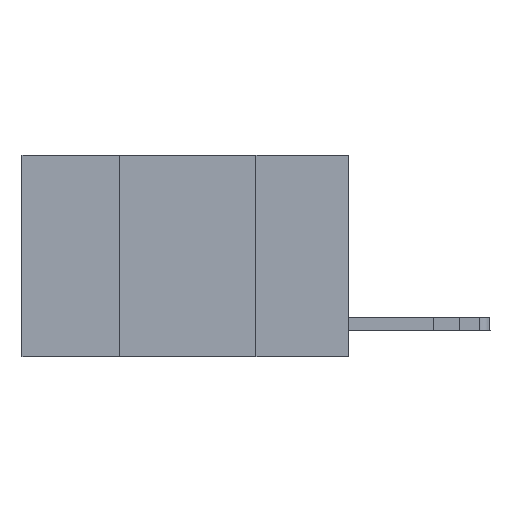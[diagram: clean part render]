
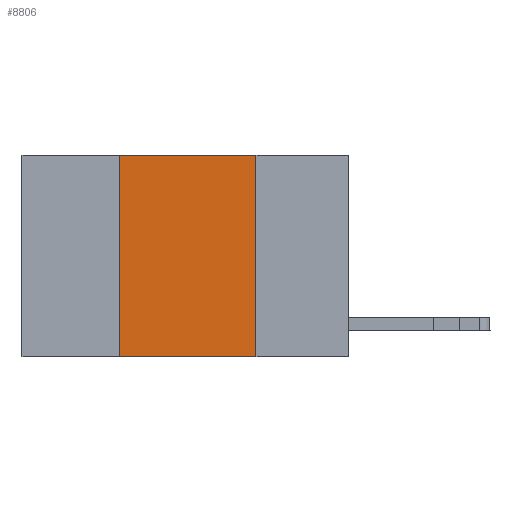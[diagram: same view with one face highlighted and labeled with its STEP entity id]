
A CAD part, left-side view. The second image highlights one B-rep face of the part: STEP entity #8806.
In plain terms, the highlighted planar face has unit normal (-1, 0, 0).
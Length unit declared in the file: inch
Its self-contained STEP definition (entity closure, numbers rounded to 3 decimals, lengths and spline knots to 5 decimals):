
#1164 = EDGE_CURVE ( 'NONE', #3525, #4443, #15752, .T. ) ;
#1372 = VECTOR ( 'NONE', #15229, 39.37008 ) ;
#1936 = LINE ( 'NONE', #8537, #1372 ) ;
#2475 = CARTESIAN_POINT ( 'NONE',  ( 0., 0.17, -0.37 ) ) ;
#3525 = VERTEX_POINT ( 'NONE', #12645 ) ;
#3609 = PLANE ( 'NONE',  #5714 ) ;
#3705 = DIRECTION ( 'NONE',  ( 1., 0., 0. ) ) ;
#3741 = CARTESIAN_POINT ( 'NONE',  ( 0., 0.17, 0. ) ) ;
#4443 = VERTEX_POINT ( 'NONE', #2475 ) ;
#5211 = VECTOR ( 'NONE', #13344, 39.37008 ) ;
#5714 = AXIS2_PLACEMENT_3D ( 'NONE', #7008, #3705, #20737 ) ;
#7008 = CARTESIAN_POINT ( 'NONE',  ( 0., 0.6, 0. ) ) ;
#7611 = ORIENTED_EDGE ( 'NONE', *, *, #21292, .F. ) ;
#7775 = DIRECTION ( 'NONE',  ( 0., -1., 0. ) ) ;
#7928 = VERTEX_POINT ( 'NONE', #10378 ) ;
#8105 = ORIENTED_EDGE ( 'NONE', *, *, #1164, .F. ) ;
#8537 = CARTESIAN_POINT ( 'NONE',  ( 0., 0.6, -0.37 ) ) ;
#8554 = FACE_OUTER_BOUND ( 'NONE', #21101, .T. ) ;
#8806 = ADVANCED_FACE ( 'NONE', ( #8554 ), #3609, .F. ) ;
#8843 = CARTESIAN_POINT ( 'NONE',  ( 0., 0.42, 0. ) ) ;
#10378 = CARTESIAN_POINT ( 'NONE',  ( 0., 0.42, -0.37 ) ) ;
#10873 = EDGE_CURVE ( 'NONE', #17776, #3525, #16117, .T. ) ;
#12645 = CARTESIAN_POINT ( 'NONE',  ( 0., 0.17, 0. ) ) ;
#13344 = DIRECTION ( 'NONE',  ( 0., 0., 1. ) ) ;
#13490 = ORIENTED_EDGE ( 'NONE', *, *, #16170, .T. ) ;
#15087 = CARTESIAN_POINT ( 'NONE',  ( 0., 0.42, 0. ) ) ;
#15229 = DIRECTION ( 'NONE',  ( 0., -1., 0. ) ) ;
#15752 = LINE ( 'NONE', #3741, #16834 ) ;
#16117 = LINE ( 'NONE', #16228, #18187 ) ;
#16170 = EDGE_CURVE ( 'NONE', #7928, #4443, #1936, .T. ) ;
#16228 = CARTESIAN_POINT ( 'NONE',  ( 0., 0.6, 0. ) ) ;
#16495 = ORIENTED_EDGE ( 'NONE', *, *, #10873, .F. ) ;
#16834 = VECTOR ( 'NONE', #20214, 39.37008 ) ;
#17776 = VERTEX_POINT ( 'NONE', #8843 ) ;
#18187 = VECTOR ( 'NONE', #7775, 39.37008 ) ;
#20214 = DIRECTION ( 'NONE',  ( 0., 0., -1. ) ) ;
#20737 = DIRECTION ( 'NONE',  ( 0., 0., -1. ) ) ;
#21101 = EDGE_LOOP ( 'NONE', ( #8105, #16495, #7611, #13490 ) ) ;
#21292 = EDGE_CURVE ( 'NONE', #7928, #17776, #21671, .T. ) ;
#21671 = LINE ( 'NONE', #15087, #5211 ) ;
